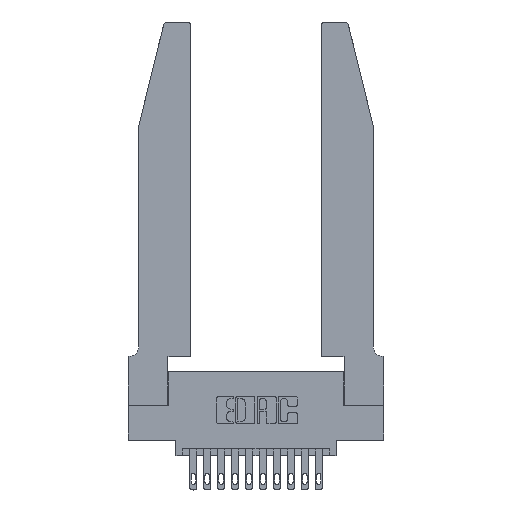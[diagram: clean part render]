
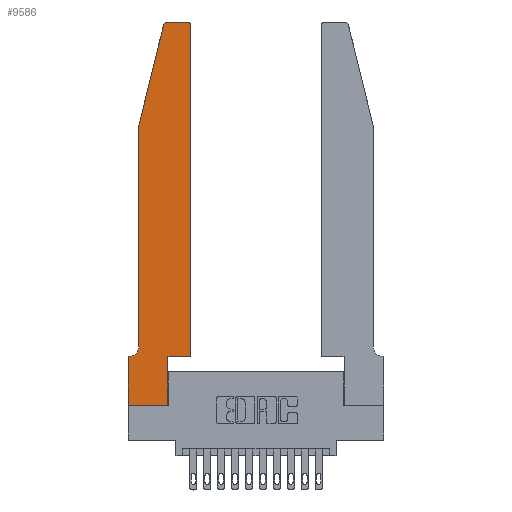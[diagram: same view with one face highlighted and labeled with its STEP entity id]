
A CAD part, top view. The second image highlights one B-rep face of the part: STEP entity #9586.
In plain terms, the highlighted planar face has unit normal (0, 0, 1).
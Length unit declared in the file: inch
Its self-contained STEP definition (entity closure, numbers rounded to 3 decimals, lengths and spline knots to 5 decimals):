
#20 = CARTESIAN_POINT ( 'NONE',  ( 0.4505, 0.35, 0.37 ) ) ;
#77 = LINE ( 'NONE', #2316, #14855 ) ;
#182 = EDGE_CURVE ( 'NONE', #9167, #5553, #3028, .T. ) ;
#205 = CARTESIAN_POINT ( 'NONE',  ( 0., 0., 0.37 ) ) ;
#304 = LINE ( 'NONE', #16043, #3591 ) ;
#1058 = DIRECTION ( 'NONE',  ( 0., 1., 0. ) ) ;
#1183 = CARTESIAN_POINT ( 'NONE',  ( 0.0755, 0.35, 0.37 ) ) ;
#1465 = VERTEX_POINT ( 'NONE', #4847 ) ;
#1673 = LINE ( 'NONE', #15435, #6179 ) ;
#1923 = CARTESIAN_POINT ( 'NONE',  ( 0., 0., 0.37 ) ) ;
#1924 = ORIENTED_EDGE ( 'NONE', *, *, #8915, .T. ) ;
#2081 = VECTOR ( 'NONE', #1058, 39.37008 ) ;
#2150 = ORIENTED_EDGE ( 'NONE', *, *, #6081, .T. ) ;
#2217 = CARTESIAN_POINT ( 'NONE',  ( 0.2865, 0.35, 0.37 ) ) ;
#2292 = EDGE_CURVE ( 'NONE', #6551, #14640, #2559, .T. ) ;
#2316 = CARTESIAN_POINT ( 'NONE',  ( 0.0755, 2., 0.37 ) ) ;
#2559 = LINE ( 'NONE', #9823, #3151 ) ;
#2644 = CARTESIAN_POINT ( 'NONE',  ( 0.284, 2.75, 0.37 ) ) ;
#2832 = DIRECTION ( 'NONE',  ( 0., 1., 0. ) ) ;
#2849 = VECTOR ( 'NONE', #2832, 39.37008 ) ;
#2854 = CARTESIAN_POINT ( 'NONE',  ( 0.2865, 0., 0.37 ) ) ;
#2935 = ORIENTED_EDGE ( 'NONE', *, *, #11791, .T. ) ;
#2956 = LINE ( 'NONE', #9092, #16907 ) ;
#3028 = LINE ( 'NONE', #1183, #11657 ) ;
#3051 = LINE ( 'NONE', #20, #2849 ) ;
#3151 = VECTOR ( 'NONE', #4629, 39.37008 ) ;
#3466 = LINE ( 'NONE', #1923, #13945 ) ;
#3591 = VECTOR ( 'NONE', #5502, 39.37008 ) ;
#3747 = ORIENTED_EDGE ( 'NONE', *, *, #15723, .T. ) ;
#3746 = CARTESIAN_POINT ( 'NONE',  ( 0.2865, 0.35, 0.37 ) ) ;
#3894 = LINE ( 'NONE', #3746, #2081 ) ;
#3962 = EDGE_CURVE ( 'NONE', #4928, #9167, #5798, .T. ) ;
#4249 = VERTEX_POINT ( 'NONE', #205 ) ;
#4261 = CARTESIAN_POINT ( 'NONE',  ( 0.0055, 0.42, 0.37 ) ) ;
#4280 = CARTESIAN_POINT ( 'NONE',  ( 0.4205, 2.72, 0.37 ) ) ;
#4346 = DIRECTION ( 'NONE',  ( 1., 0., 0. ) ) ;
#4629 = DIRECTION ( 'NONE',  ( -1., 0., 0. ) ) ;
#4847 = CARTESIAN_POINT ( 'NONE',  ( 0.4505, 2.72, 0.37 ) ) ;
#4928 = VERTEX_POINT ( 'NONE', #10400 ) ;
#5395 = CARTESIAN_POINT ( 'NONE',  ( 0.0055, 0.35, 0.37 ) ) ;
#5502 = DIRECTION ( 'NONE',  ( 0., -1., 0. ) ) ;
#5553 = VERTEX_POINT ( 'NONE', #8333 ) ;
#5733 = DIRECTION ( 'NONE',  ( 0., 0., 1. ) ) ;
#5751 = DIRECTION ( 'NONE',  ( -1., 0., 0. ) ) ;
#5798 = CIRCLE ( 'NONE', #6661, 0.07 ) ;
#5805 = ORIENTED_EDGE ( 'NONE', *, *, #2292, .T. ) ;
#6081 = EDGE_CURVE ( 'NONE', #13822, #1465, #3051, .T. ) ;
#6179 = VECTOR ( 'NONE', #8926, 39.37008 ) ;
#6235 = VERTEX_POINT ( 'NONE', #2217 ) ;
#6414 = DIRECTION ( 'NONE',  ( 1., 0., 0. ) ) ;
#6492 = DIRECTION ( 'NONE',  ( 0., 0., 1. ) ) ;
#6525 = PLANE ( 'NONE',  #8563 ) ;
#6551 = VERTEX_POINT ( 'NONE', #11078 ) ;
#6661 = AXIS2_PLACEMENT_3D ( 'NONE', #4261, #12272, #5751 ) ;
#6670 = FACE_OUTER_BOUND ( 'NONE', #10214, .T. ) ;
#6732 = VERTEX_POINT ( 'NONE', #7553 ) ;
#6896 = EDGE_CURVE ( 'NONE', #4249, #13392, #3466, .T. ) ;
#7553 = CARTESIAN_POINT ( 'NONE',  ( 0.25487, 2.72718, 0.37 ) ) ;
#7935 = ORIENTED_EDGE ( 'NONE', *, *, #182, .T. ) ;
#8333 = CARTESIAN_POINT ( 'NONE',  ( 0., 0.35, 0.37 ) ) ;
#8364 = ORIENTED_EDGE ( 'NONE', *, *, #9306, .T. ) ;
#8563 = AXIS2_PLACEMENT_3D ( 'NONE', #15638, #11561, #6414 ) ;
#8661 = ORIENTED_EDGE ( 'NONE', *, *, #13295, .T. ) ;
#8792 = ORIENTED_EDGE ( 'NONE', *, *, #6896, .T. ) ;
#8915 = EDGE_CURVE ( 'NONE', #14640, #6732, #11392, .T. ) ;
#8926 = DIRECTION ( 'NONE',  ( 1., 0., 0. ) ) ;
#9092 = CARTESIAN_POINT ( 'NONE',  ( 0.0755, 2., 0.37 ) ) ;
#9167 = VERTEX_POINT ( 'NONE', #5395 ) ;
#9306 = EDGE_CURVE ( 'NONE', #5553, #4249, #304, .T. ) ;
#9586 = ADVANCED_FACE ( 'NONE', ( #6670 ), #6525, .T. ) ;
#9652 = AXIS2_PLACEMENT_3D ( 'NONE', #10250, #6492, #10372 ) ;
#9823 = CARTESIAN_POINT ( 'NONE',  ( 0.2605, 2.75, 0.37 ) ) ;
#9910 = VERTEX_POINT ( 'NONE', #12475 ) ;
#10013 = EDGE_CURVE ( 'NONE', #9910, #4928, #77, .T. ) ;
#10214 = EDGE_LOOP ( 'NONE', ( #5805, #1924, #8661, #11508, #12313, #7935, #8364, #8792, #3747, #2935, #2150, #13738 ) ) ;
#10250 = CARTESIAN_POINT ( 'NONE',  ( 0.284, 2.72, 0.37 ) ) ;
#10356 = AXIS2_PLACEMENT_3D ( 'NONE', #4280, #5733, #4346 ) ;
#10372 = DIRECTION ( 'NONE',  ( 1., 0., 0. ) ) ;
#10400 = CARTESIAN_POINT ( 'NONE',  ( 0.0755, 0.42, 0.37 ) ) ;
#10423 = DIRECTION ( 'NONE',  ( -0.239, -0.971, 0. ) ) ;
#10813 = DIRECTION ( 'NONE',  ( 1., 0., 0. ) ) ;
#11078 = CARTESIAN_POINT ( 'NONE',  ( 0.4205, 2.75, 0.37 ) ) ;
#11392 = CIRCLE ( 'NONE', #9652, 0.03 ) ;
#11508 = ORIENTED_EDGE ( 'NONE', *, *, #10013, .T. ) ;
#11561 = DIRECTION ( 'NONE',  ( 0., 0., 1. ) ) ;
#11657 = VECTOR ( 'NONE', #13668, 39.37008 ) ;
#11791 = EDGE_CURVE ( 'NONE', #6235, #13822, #1673, .T. ) ;
#12272 = DIRECTION ( 'NONE',  ( 0., 0., -1. ) ) ;
#12313 = ORIENTED_EDGE ( 'NONE', *, *, #3962, .T. ) ;
#12475 = CARTESIAN_POINT ( 'NONE',  ( 0.0755, 2., 0.37 ) ) ;
#12851 = DIRECTION ( 'NONE',  ( 0., -1., 0. ) ) ;
#13295 = EDGE_CURVE ( 'NONE', #6732, #9910, #2956, .T. ) ;
#13392 = VERTEX_POINT ( 'NONE', #2854 ) ;
#13668 = DIRECTION ( 'NONE',  ( -1., 0., 0. ) ) ;
#13738 = ORIENTED_EDGE ( 'NONE', *, *, #15426, .T. ) ;
#13822 = VERTEX_POINT ( 'NONE', #16666 ) ;
#13945 = VECTOR ( 'NONE', #10813, 39.37008 ) ;
#14640 = VERTEX_POINT ( 'NONE', #2644 ) ;
#14855 = VECTOR ( 'NONE', #12851, 39.37008 ) ;
#15426 = EDGE_CURVE ( 'NONE', #1465, #6551, #16217, .T. ) ;
#15435 = CARTESIAN_POINT ( 'NONE',  ( 0.4505, 0.35, 0.37 ) ) ;
#15638 = CARTESIAN_POINT ( 'NONE',  ( 0., 0.35, 0.37 ) ) ;
#15723 = EDGE_CURVE ( 'NONE', #13392, #6235, #3894, .T. ) ;
#16043 = CARTESIAN_POINT ( 'NONE',  ( 0., 0., 0.37 ) ) ;
#16217 = CIRCLE ( 'NONE', #10356, 0.03 ) ;
#16666 = CARTESIAN_POINT ( 'NONE',  ( 0.4505, 0.35, 0.37 ) ) ;
#16907 = VECTOR ( 'NONE', #10423, 39.37008 ) ;
